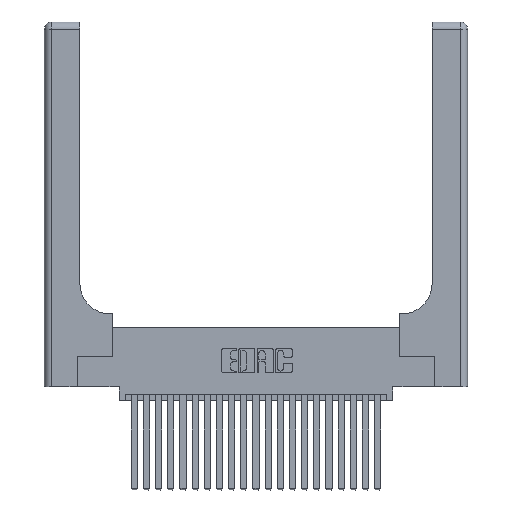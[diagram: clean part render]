
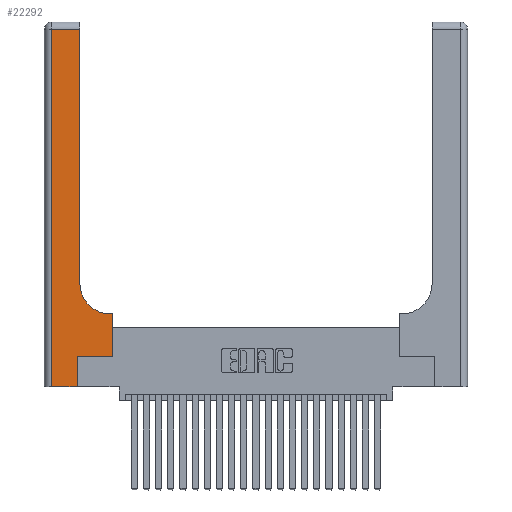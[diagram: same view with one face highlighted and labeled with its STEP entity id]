
A CAD part, top view. The second image highlights one B-rep face of the part: STEP entity #22292.
In plain terms, the highlighted planar face has unit normal (0, 0, 1).
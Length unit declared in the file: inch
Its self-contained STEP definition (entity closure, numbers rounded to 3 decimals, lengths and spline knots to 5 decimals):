
#720 = DIRECTION ( 'NONE',  ( 0., 0., -1. ) ) ;
#1423 = PLANE ( 'NONE',  #19706 ) ;
#1500 = VECTOR ( 'NONE', #5180, 39.37008 ) ;
#1814 = VERTEX_POINT ( 'NONE', #17039 ) ;
#1906 = VERTEX_POINT ( 'NONE', #22594 ) ;
#2029 = EDGE_CURVE ( 'NONE', #1906, #23867, #3387, .T. ) ;
#2275 = EDGE_CURVE ( 'NONE', #1814, #20408, #12790, .T. ) ;
#2534 = VERTEX_POINT ( 'NONE', #19045 ) ;
#2600 = VECTOR ( 'NONE', #15097, 39.37008 ) ;
#2608 = CARTESIAN_POINT ( 'NONE',  ( 0.5585, 0.6, 0.37 ) ) ;
#2702 = EDGE_CURVE ( 'NONE', #23867, #12996, #9508, .T. ) ;
#3032 = ORIENTED_EDGE ( 'NONE', *, *, #9859, .T. ) ;
#3042 = EDGE_CURVE ( 'NONE', #23552, #23604, #8019, .T. ) ;
#3387 = LINE ( 'NONE', #10528, #23238 ) ;
#3422 = VERTEX_POINT ( 'NONE', #22923 ) ;
#4305 = ORIENTED_EDGE ( 'NONE', *, *, #3042, .T. ) ;
#5180 = DIRECTION ( 'NONE',  ( 0., -1., 0. ) ) ;
#5363 = ORIENTED_EDGE ( 'NONE', *, *, #15050, .T. ) ;
#5493 = DIRECTION ( 'NONE',  ( -1., 0., 0. ) ) ;
#5552 = CARTESIAN_POINT ( 'NONE',  ( 0., 3., 0.37 ) ) ;
#5902 = LINE ( 'NONE', #23447, #19571 ) ;
#5936 = DIRECTION ( 'NONE',  ( 0., 1., 0. ) ) ;
#7505 = DIRECTION ( 'NONE',  ( -1., 0., 0. ) ) ;
#7636 = CARTESIAN_POINT ( 'NONE',  ( 0.269, 0., 0.37 ) ) ;
#7745 = VECTOR ( 'NONE', #23818, 39.37008 ) ;
#8019 = LINE ( 'NONE', #13066, #17901 ) ;
#8686 = ORIENTED_EDGE ( 'NONE', *, *, #16661, .T. ) ;
#8789 = ORIENTED_EDGE ( 'NONE', *, *, #12303, .T. ) ;
#9508 = LINE ( 'NONE', #17647, #13897 ) ;
#9859 = EDGE_CURVE ( 'NONE', #23604, #1814, #11973, .T. ) ;
#10131 = LINE ( 'NONE', #17074, #14466 ) ;
#10528 = CARTESIAN_POINT ( 'NONE',  ( 0.5585, 0.25, 0.37 ) ) ;
#11308 = CIRCLE ( 'NONE', #17522, 0.25 ) ;
#11324 = ORIENTED_EDGE ( 'NONE', *, *, #2029, .T. ) ;
#11409 = CARTESIAN_POINT ( 'NONE',  ( 0.2915, 2.94, 0.37 ) ) ;
#11973 = LINE ( 'NONE', #18296, #1500 ) ;
#12303 = EDGE_CURVE ( 'NONE', #3422, #1906, #5902, .T. ) ;
#12509 = CARTESIAN_POINT ( 'NONE',  ( 0.5415, 0.85, 0.37 ) ) ;
#12790 = LINE ( 'NONE', #22028, #7745 ) ;
#12996 = VERTEX_POINT ( 'NONE', #19988 ) ;
#13066 = CARTESIAN_POINT ( 'NONE',  ( 0., 2.94, 0.37 ) ) ;
#13897 = VECTOR ( 'NONE', #17730, 39.37008 ) ;
#14067 = ORIENTED_EDGE ( 'NONE', *, *, #2275, .T. ) ;
#14341 = DIRECTION ( 'NONE',  ( 1., 0., 0. ) ) ;
#14466 = VECTOR ( 'NONE', #5936, 39.37008 ) ;
#14474 = DIRECTION ( 'NONE',  ( 1., 0., 0. ) ) ;
#15050 = EDGE_CURVE ( 'NONE', #2534, #23552, #10131, .T. ) ;
#15097 = DIRECTION ( 'NONE',  ( 0., 1., 0. ) ) ;
#15345 = EDGE_CURVE ( 'NONE', #12996, #2534, #11308, .T. ) ;
#16661 = EDGE_CURVE ( 'NONE', #20408, #3422, #22557, .T. ) ;
#17039 = CARTESIAN_POINT ( 'NONE',  ( 0.06, 0., 0.37 ) ) ;
#17074 = CARTESIAN_POINT ( 'NONE',  ( 0.2915, 3., 0.37 ) ) ;
#17522 = AXIS2_PLACEMENT_3D ( 'NONE', #12509, #720, #14341 ) ;
#17647 = CARTESIAN_POINT ( 'NONE',  ( 0.2915, 0.6, 0.37 ) ) ;
#17712 = FACE_OUTER_BOUND ( 'NONE', #22255, .T. ) ;
#17730 = DIRECTION ( 'NONE',  ( -1., 0., 0. ) ) ;
#17901 = VECTOR ( 'NONE', #5493, 39.37008 ) ;
#18296 = CARTESIAN_POINT ( 'NONE',  ( 0.06, 3., 0.37 ) ) ;
#18618 = DIRECTION ( 'NONE',  ( 0., 0., -1. ) ) ;
#19045 = CARTESIAN_POINT ( 'NONE',  ( 0.2915, 0.85, 0.37 ) ) ;
#19571 = VECTOR ( 'NONE', #14474, 39.37008 ) ;
#19706 = AXIS2_PLACEMENT_3D ( 'NONE', #5552, #18618, #7505 ) ;
#19980 = ORIENTED_EDGE ( 'NONE', *, *, #2702, .T. ) ;
#19988 = CARTESIAN_POINT ( 'NONE',  ( 0.5415, 0.6, 0.37 ) ) ;
#20408 = VERTEX_POINT ( 'NONE', #7636 ) ;
#20761 = CARTESIAN_POINT ( 'NONE',  ( 0.06, 2.94, 0.37 ) ) ;
#21235 = ORIENTED_EDGE ( 'NONE', *, *, #15345, .T. ) ;
#22028 = CARTESIAN_POINT ( 'NONE',  ( 0., 0., 0.37 ) ) ;
#22255 = EDGE_LOOP ( 'NONE', ( #5363, #4305, #3032, #14067, #8686, #8789, #11324, #19980, #21235 ) ) ;
#22292 = ADVANCED_FACE ( 'NONE', ( #17712 ), #1423, .F. ) ;
#22557 = LINE ( 'NONE', #24045, #2600 ) ;
#22594 = CARTESIAN_POINT ( 'NONE',  ( 0.5585, 0.25, 0.37 ) ) ;
#22923 = CARTESIAN_POINT ( 'NONE',  ( 0.269, 0.25, 0.37 ) ) ;
#23211 = DIRECTION ( 'NONE',  ( 0., 1., 0. ) ) ;
#23238 = VECTOR ( 'NONE', #23211, 39.37008 ) ;
#23447 = CARTESIAN_POINT ( 'NONE',  ( 0.269, 0.25, 0.37 ) ) ;
#23552 = VERTEX_POINT ( 'NONE', #11409 ) ;
#23604 = VERTEX_POINT ( 'NONE', #20761 ) ;
#23818 = DIRECTION ( 'NONE',  ( 1., 0., 0. ) ) ;
#23867 = VERTEX_POINT ( 'NONE', #2608 ) ;
#24045 = CARTESIAN_POINT ( 'NONE',  ( 0.269, 0., 0.37 ) ) ;
